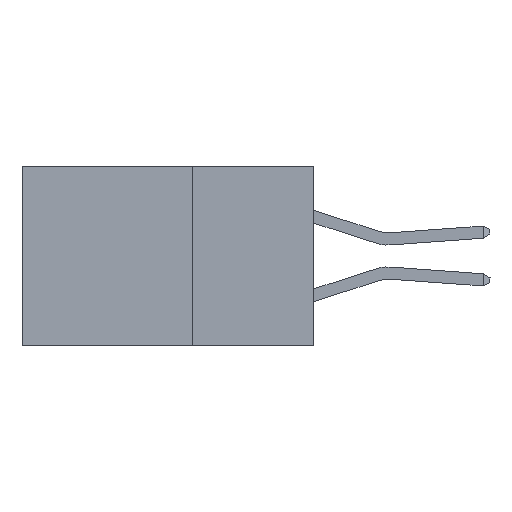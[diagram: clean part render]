
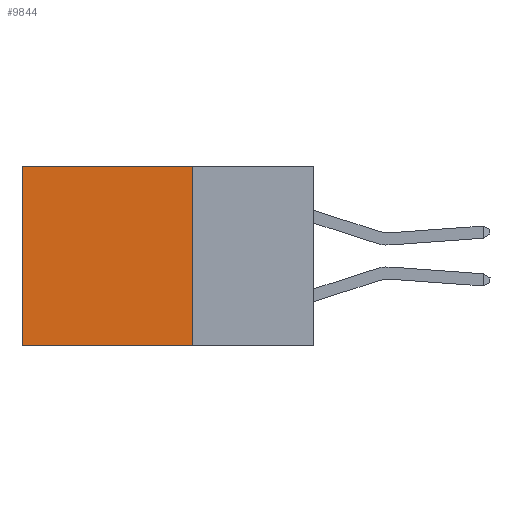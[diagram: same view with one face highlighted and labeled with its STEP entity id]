
A CAD part, left-side view. The second image highlights one B-rep face of the part: STEP entity #9844.
In plain terms, the highlighted planar face has unit normal (-1, 0, 0).
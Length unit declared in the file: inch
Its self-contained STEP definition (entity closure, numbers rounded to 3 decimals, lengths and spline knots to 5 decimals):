
#389 = CARTESIAN_POINT ( 'NONE',  ( 0.2875, 0.25, -0.37 ) ) ;
#1269 = EDGE_CURVE ( 'NONE', #18552, #17510, #7794, .T. ) ;
#1985 = CARTESIAN_POINT ( 'NONE',  ( 0.2875, 0.25, 0. ) ) ;
#2200 = EDGE_CURVE ( 'NONE', #18029, #18552, #20760, .T. ) ;
#2440 = EDGE_CURVE ( 'NONE', #18029, #11246, #11521, .T. ) ;
#2725 = VECTOR ( 'NONE', #19902, 39.37008 ) ;
#4186 = ORIENTED_EDGE ( 'NONE', *, *, #13920, .T. ) ;
#4858 = FACE_OUTER_BOUND ( 'NONE', #16491, .T. ) ;
#6617 = ORIENTED_EDGE ( 'NONE', *, *, #2440, .T. ) ;
#6887 = VECTOR ( 'NONE', #8681, 39.37008 ) ;
#7178 = DIRECTION ( 'NONE',  ( 0., 0., -1. ) ) ;
#7794 = LINE ( 'NONE', #389, #16929 ) ;
#8012 = CARTESIAN_POINT ( 'NONE',  ( 0.2875, 0.25, 0. ) ) ;
#8681 = DIRECTION ( 'NONE',  ( 0., 0., -1. ) ) ;
#9844 = ADVANCED_FACE ( 'NONE', ( #4858 ), #12352, .F. ) ;
#11055 = DIRECTION ( 'NONE',  ( 0., 1., 0. ) ) ;
#11246 = VERTEX_POINT ( 'NONE', #12138 ) ;
#11521 = LINE ( 'NONE', #20620, #21002 ) ;
#12138 = CARTESIAN_POINT ( 'NONE',  ( 0.2875, 0.6, 0. ) ) ;
#12226 = DIRECTION ( 'NONE',  ( 0., 1., 0. ) ) ;
#12352 = PLANE ( 'NONE',  #15552 ) ;
#13920 = EDGE_CURVE ( 'NONE', #11246, #17510, #20483, .T. ) ;
#14052 = CARTESIAN_POINT ( 'NONE',  ( 0.2875, 0.25, 0. ) ) ;
#15552 = AXIS2_PLACEMENT_3D ( 'NONE', #14052, #17478, #7178 ) ;
#15735 = ORIENTED_EDGE ( 'NONE', *, *, #1269, .F. ) ;
#16359 = ORIENTED_EDGE ( 'NONE', *, *, #2200, .F. ) ;
#16491 = EDGE_LOOP ( 'NONE', ( #4186, #15735, #16359, #6617 ) ) ;
#16929 = VECTOR ( 'NONE', #11055, 39.37008 ) ;
#17212 = CARTESIAN_POINT ( 'NONE',  ( 0.2875, 0.6, 0. ) ) ;
#17478 = DIRECTION ( 'NONE',  ( 1., 0., 0. ) ) ;
#17510 = VERTEX_POINT ( 'NONE', #19330 ) ;
#18029 = VERTEX_POINT ( 'NONE', #1985 ) ;
#18552 = VERTEX_POINT ( 'NONE', #18556 ) ;
#18556 = CARTESIAN_POINT ( 'NONE',  ( 0.2875, 0.25, -0.37 ) ) ;
#19330 = CARTESIAN_POINT ( 'NONE',  ( 0.2875, 0.6, -0.37 ) ) ;
#19902 = DIRECTION ( 'NONE',  ( 0., 0., -1. ) ) ;
#20483 = LINE ( 'NONE', #17212, #6887 ) ;
#20620 = CARTESIAN_POINT ( 'NONE',  ( 0.2875, 0.25, 0. ) ) ;
#20760 = LINE ( 'NONE', #8012, #2725 ) ;
#21002 = VECTOR ( 'NONE', #12226, 39.37008 ) ;
